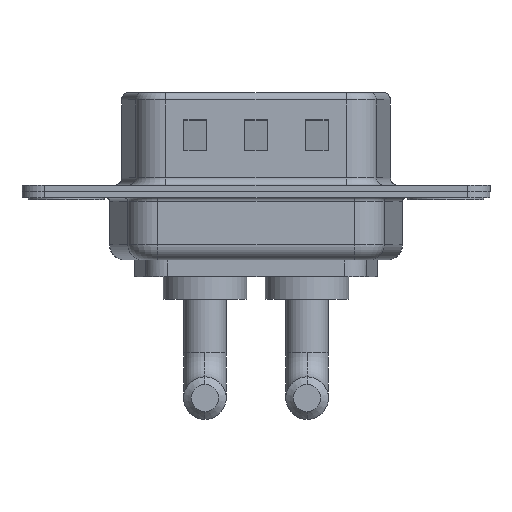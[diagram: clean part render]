
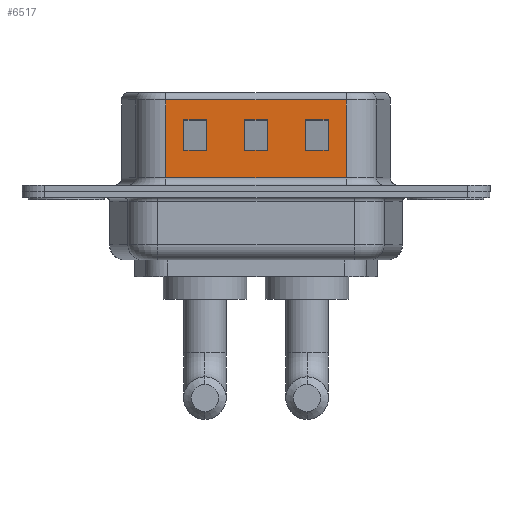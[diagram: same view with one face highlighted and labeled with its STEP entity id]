
A CAD part, front view. The second image highlights one B-rep face of the part: STEP entity #6517.
In plain terms, the highlighted planar face has unit normal (0, -1, 0).
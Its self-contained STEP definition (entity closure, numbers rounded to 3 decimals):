
#7 = EDGE_CURVE ( 'NONE', #12041, #1922, #9308, .T. ) ;
#44 = CARTESIAN_POINT ( 'NONE',  ( 6.549, -4.55, 6.02 ) ) ;
#163 = LINE ( 'NONE', #4038, #8127 ) ;
#188 = CARTESIAN_POINT ( 'NONE',  ( 9.25, -4.55, 2.705 ) ) ;
#221 = VECTOR ( 'NONE', #1267, 1000. ) ;
#238 = CARTESIAN_POINT ( 'NONE',  ( 9.25, -4.55, 6.52 ) ) ;
#456 = CARTESIAN_POINT ( 'NONE',  ( 17.25, -4.55, 4.705 ) ) ;
#504 = ORIENTED_EDGE ( 'NONE', *, *, #3896, .T. ) ;
#625 = EDGE_CURVE ( 'NONE', #1922, #3002, #3912, .T. ) ;
#639 = DIRECTION ( 'NONE',  ( -1., 0., 0. ) ) ;
#709 = ORIENTED_EDGE ( 'NONE', *, *, #1026, .T. ) ;
#761 = EDGE_LOOP ( 'NONE', ( #9744, #8204, #11528, #5645 ) ) ;
#808 = VERTEX_POINT ( 'NONE', #966 ) ;
#836 = VECTOR ( 'NONE', #1125, 1000. ) ;
#966 = CARTESIAN_POINT ( 'NONE',  ( 9.25, -4.55, 4.705 ) ) ;
#1026 = EDGE_CURVE ( 'NONE', #4444, #10832, #2283, .T. ) ;
#1104 = ORIENTED_EDGE ( 'NONE', *, *, #4622, .T. ) ;
#1125 = DIRECTION ( 'NONE',  ( 0., 0., 1. ) ) ;
#1170 = FACE_OUTER_BOUND ( 'NONE', #5575, .T. ) ;
#1190 = DIRECTION ( 'NONE',  ( 1., 0., 0. ) ) ;
#1267 = DIRECTION ( 'NONE',  ( 0., 0., 1. ) ) ;
#1361 = EDGE_CURVE ( 'NONE', #9397, #9163, #163, .T. ) ;
#1391 = ORIENTED_EDGE ( 'NONE', *, *, #5297, .F. ) ;
#1411 = DIRECTION ( 'NONE',  ( -1., 0., 0. ) ) ;
#1451 = LINE ( 'NONE', #238, #6767 ) ;
#1623 = ORIENTED_EDGE ( 'NONE', *, *, #7966, .T. ) ;
#1633 = ORIENTED_EDGE ( 'NONE', *, *, #6698, .T. ) ;
#1665 = EDGE_CURVE ( 'NONE', #9668, #4444, #1695, .T. ) ;
#1695 = LINE ( 'NONE', #5484, #5464 ) ;
#1837 = CARTESIAN_POINT ( 'NONE',  ( 14.451, -4.55, 2.705 ) ) ;
#1856 = DIRECTION ( 'NONE',  ( 0., 0., -1. ) ) ;
#1922 = VERTEX_POINT ( 'NONE', #10814 ) ;
#1937 = VERTEX_POINT ( 'NONE', #10167 ) ;
#2076 = DIRECTION ( 'NONE',  ( 0., 0., 1. ) ) ;
#2119 = PLANE ( 'NONE',  #3385 ) ;
#2176 = FACE_BOUND ( 'NONE', #7307, .T. ) ;
#2219 = CARTESIAN_POINT ( 'NONE',  ( 13.25, -4.55, 4.705 ) ) ;
#2225 = VECTOR ( 'NONE', #639, 1000. ) ;
#2228 = CARTESIAN_POINT ( 'NONE',  ( 14.451, -4.55, 4.705 ) ) ;
#2283 = LINE ( 'NONE', #9828, #221 ) ;
#2313 = CARTESIAN_POINT ( 'NONE',  ( 13.25, -4.55, 6.52 ) ) ;
#2357 = CARTESIAN_POINT ( 'NONE',  ( 15.75, -4.55, 2.705 ) ) ;
#2391 = VERTEX_POINT ( 'NONE', #11297 ) ;
#2670 = CARTESIAN_POINT ( 'NONE',  ( 18.451, -4.55, 6.52 ) ) ;
#2711 = VECTOR ( 'NONE', #1856, 1000. ) ;
#2769 = VERTEX_POINT ( 'NONE', #456 ) ;
#2804 = CARTESIAN_POINT ( 'NONE',  ( 6.549, -4.55, 6.52 ) ) ;
#2827 = LINE ( 'NONE', #11718, #10273 ) ;
#3002 = VERTEX_POINT ( 'NONE', #9056 ) ;
#3134 = CARTESIAN_POINT ( 'NONE',  ( 18.451, -4.55, 6.02 ) ) ;
#3198 = LINE ( 'NONE', #10926, #5604 ) ;
#3261 = LINE ( 'NONE', #3134, #5063 ) ;
#3272 = DIRECTION ( 'NONE',  ( 0., 0., -1. ) ) ;
#3385 = AXIS2_PLACEMENT_3D ( 'NONE', #9973, #6865, #4968 ) ;
#3780 = CARTESIAN_POINT ( 'NONE',  ( 7.75, -4.55, 6.52 ) ) ;
#3896 = EDGE_CURVE ( 'NONE', #9163, #10996, #11962, .T. ) ;
#3912 = LINE ( 'NONE', #3780, #836 ) ;
#3917 = VECTOR ( 'NONE', #3272, 1000. ) ;
#4038 = CARTESIAN_POINT ( 'NONE',  ( 18.451, -4.55, 4.705 ) ) ;
#4116 = CARTESIAN_POINT ( 'NONE',  ( 17.25, -4.55, 6.52 ) ) ;
#4138 = CARTESIAN_POINT ( 'NONE',  ( 18.451, -4.55, 6.02 ) ) ;
#4199 = CARTESIAN_POINT ( 'NONE',  ( 15.75, -4.55, 4.705 ) ) ;
#4335 = CARTESIAN_POINT ( 'NONE',  ( 18.451, -4.55, 2.705 ) ) ;
#4366 = VERTEX_POINT ( 'NONE', #4138 ) ;
#4444 = VERTEX_POINT ( 'NONE', #2357 ) ;
#4507 = DIRECTION ( 'NONE',  ( 0., 0., -1. ) ) ;
#4554 = VECTOR ( 'NONE', #4507, 1000. ) ;
#4622 = EDGE_CURVE ( 'NONE', #10989, #1937, #6654, .T. ) ;
#4827 = EDGE_CURVE ( 'NONE', #808, #12041, #1451, .T. ) ;
#4968 = DIRECTION ( 'NONE',  ( -1., 0., 0. ) ) ;
#5063 = VECTOR ( 'NONE', #1411, 1000. ) ;
#5149 = FACE_BOUND ( 'NONE', #8102, .T. ) ;
#5188 = ORIENTED_EDGE ( 'NONE', *, *, #11606, .T. ) ;
#5198 = LINE ( 'NONE', #2228, #12502 ) ;
#5297 = EDGE_CURVE ( 'NONE', #4366, #6522, #11370, .T. ) ;
#5307 = DIRECTION ( 'NONE',  ( 0., 0., -1. ) ) ;
#5339 = LINE ( 'NONE', #4335, #5603 ) ;
#5355 = ORIENTED_EDGE ( 'NONE', *, *, #1665, .T. ) ;
#5464 = VECTOR ( 'NONE', #10637, 1000. ) ;
#5484 = CARTESIAN_POINT ( 'NONE',  ( 22.451, -4.55, 2.705 ) ) ;
#5575 = EDGE_LOOP ( 'NONE', ( #1391, #5188, #1104, #7725 ) ) ;
#5603 = VECTOR ( 'NONE', #8069, 1000. ) ;
#5604 = VECTOR ( 'NONE', #12084, 1000. ) ;
#5645 = ORIENTED_EDGE ( 'NONE', *, *, #7052, .T. ) ;
#5681 = ORIENTED_EDGE ( 'NONE', *, *, #5710, .T. ) ;
#5710 = EDGE_CURVE ( 'NONE', #2769, #9668, #10895, .T. ) ;
#6001 = CARTESIAN_POINT ( 'NONE',  ( 11.75, -4.55, 4.705 ) ) ;
#6185 = DIRECTION ( 'NONE',  ( 0., 0., -1. ) ) ;
#6517 = ADVANCED_FACE ( 'NONE', ( #8781, #5149, #2176, #1170 ), #2119, .F. ) ;
#6522 = VERTEX_POINT ( 'NONE', #6993 ) ;
#6654 = LINE ( 'NONE', #2804, #2711 ) ;
#6698 = EDGE_CURVE ( 'NONE', #10996, #2391, #5339, .T. ) ;
#6699 = ORIENTED_EDGE ( 'NONE', *, *, #1361, .T. ) ;
#6767 = VECTOR ( 'NONE', #5307, 1000. ) ;
#6865 = DIRECTION ( 'NONE',  ( 0., 1., 0. ) ) ;
#6879 = CARTESIAN_POINT ( 'NONE',  ( 13.25, -4.55, 2.705 ) ) ;
#6993 = CARTESIAN_POINT ( 'NONE',  ( 18.451, -4.55, 0.9 ) ) ;
#7052 = EDGE_CURVE ( 'NONE', #3002, #808, #5198, .T. ) ;
#7307 = EDGE_LOOP ( 'NONE', ( #6699, #504, #1633, #8927 ) ) ;
#7725 = ORIENTED_EDGE ( 'NONE', *, *, #7839, .T. ) ;
#7837 = LINE ( 'NONE', #11727, #8889 ) ;
#7839 = EDGE_CURVE ( 'NONE', #1937, #6522, #2827, .T. ) ;
#7966 = EDGE_CURVE ( 'NONE', #10832, #2769, #3198, .T. ) ;
#7977 = CARTESIAN_POINT ( 'NONE',  ( 17.25, -4.55, 2.705 ) ) ;
#8069 = DIRECTION ( 'NONE',  ( -1., 0., 0. ) ) ;
#8102 = EDGE_LOOP ( 'NONE', ( #5681, #5355, #709, #1623 ) ) ;
#8127 = VECTOR ( 'NONE', #1190, 1000. ) ;
#8204 = ORIENTED_EDGE ( 'NONE', *, *, #7, .T. ) ;
#8407 = VECTOR ( 'NONE', #6185, 1000. ) ;
#8781 = FACE_BOUND ( 'NONE', #761, .T. ) ;
#8889 = VECTOR ( 'NONE', #2076, 1000. ) ;
#8927 = ORIENTED_EDGE ( 'NONE', *, *, #11088, .T. ) ;
#9056 = CARTESIAN_POINT ( 'NONE',  ( 7.75, -4.55, 4.705 ) ) ;
#9163 = VERTEX_POINT ( 'NONE', #2219 ) ;
#9308 = LINE ( 'NONE', #1837, #2225 ) ;
#9397 = VERTEX_POINT ( 'NONE', #6001 ) ;
#9668 = VERTEX_POINT ( 'NONE', #7977 ) ;
#9744 = ORIENTED_EDGE ( 'NONE', *, *, #4827, .T. ) ;
#9828 = CARTESIAN_POINT ( 'NONE',  ( 15.75, -4.55, 6.52 ) ) ;
#9973 = CARTESIAN_POINT ( 'NONE',  ( 18.451, -4.55, 6.52 ) ) ;
#10167 = CARTESIAN_POINT ( 'NONE',  ( 6.549, -4.55, 0.9 ) ) ;
#10273 = VECTOR ( 'NONE', #11662, 1000. ) ;
#10637 = DIRECTION ( 'NONE',  ( -1., 0., 0. ) ) ;
#10814 = CARTESIAN_POINT ( 'NONE',  ( 7.75, -4.55, 2.705 ) ) ;
#10832 = VERTEX_POINT ( 'NONE', #4199 ) ;
#10895 = LINE ( 'NONE', #4116, #8407 ) ;
#10912 = DIRECTION ( 'NONE',  ( 1., 0., 0. ) ) ;
#10926 = CARTESIAN_POINT ( 'NONE',  ( 22.451, -4.55, 4.705 ) ) ;
#10989 = VERTEX_POINT ( 'NONE', #44 ) ;
#10996 = VERTEX_POINT ( 'NONE', #6879 ) ;
#11088 = EDGE_CURVE ( 'NONE', #2391, #9397, #7837, .T. ) ;
#11297 = CARTESIAN_POINT ( 'NONE',  ( 11.75, -4.55, 2.705 ) ) ;
#11370 = LINE ( 'NONE', #2670, #4554 ) ;
#11528 = ORIENTED_EDGE ( 'NONE', *, *, #625, .T. ) ;
#11606 = EDGE_CURVE ( 'NONE', #4366, #10989, #3261, .T. ) ;
#11662 = DIRECTION ( 'NONE',  ( 1., 0., 0. ) ) ;
#11718 = CARTESIAN_POINT ( 'NONE',  ( 18.451, -4.55, 0.9 ) ) ;
#11727 = CARTESIAN_POINT ( 'NONE',  ( 11.75, -4.55, 6.52 ) ) ;
#11962 = LINE ( 'NONE', #2313, #3917 ) ;
#12041 = VERTEX_POINT ( 'NONE', #188 ) ;
#12084 = DIRECTION ( 'NONE',  ( 1., 0., 0. ) ) ;
#12502 = VECTOR ( 'NONE', #10912, 1000. ) ;
